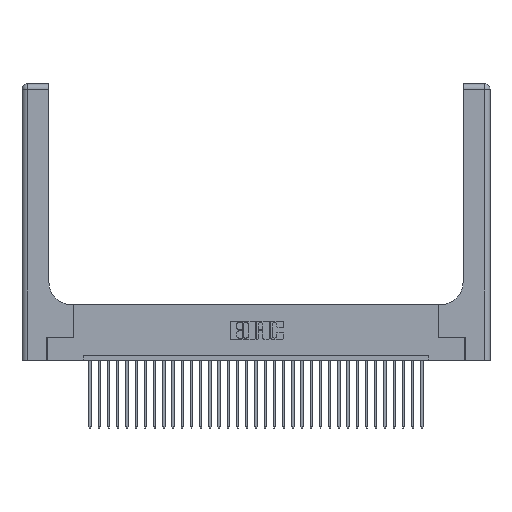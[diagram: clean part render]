
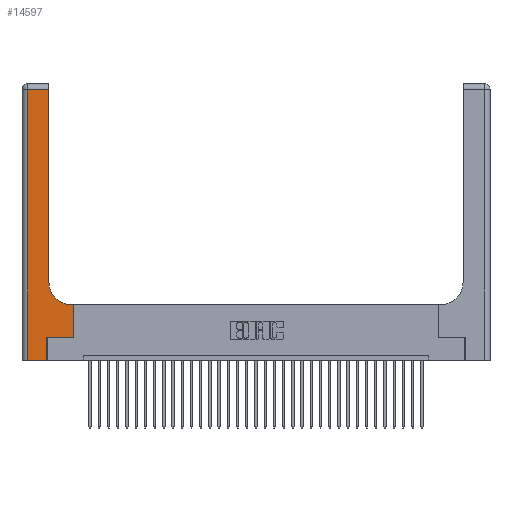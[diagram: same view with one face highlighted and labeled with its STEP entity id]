
A CAD part, top view. The second image highlights one B-rep face of the part: STEP entity #14597.
In plain terms, the highlighted planar face has unit normal (0, 0, 1).
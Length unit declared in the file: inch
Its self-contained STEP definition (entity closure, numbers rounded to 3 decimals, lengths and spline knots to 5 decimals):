
#437 = CARTESIAN_POINT ( 'NONE',  ( 0.2915, 2.94, 0.37 ) ) ;
#638 = LINE ( 'NONE', #29766, #29115 ) ;
#1435 = CARTESIAN_POINT ( 'NONE',  ( 0.269, 0., 0.37 ) ) ;
#1595 = CARTESIAN_POINT ( 'NONE',  ( 0.06, 3., 0.37 ) ) ;
#2507 = CARTESIAN_POINT ( 'NONE',  ( 0.5585, 0.25, 0.37 ) ) ;
#3038 = LINE ( 'NONE', #1595, #9125 ) ;
#3089 = CARTESIAN_POINT ( 'NONE',  ( 0.2915, 0.85, 0.37 ) ) ;
#4243 = CARTESIAN_POINT ( 'NONE',  ( 0., 2.94, 0.37 ) ) ;
#4398 = DIRECTION ( 'NONE',  ( 0., -1., 0. ) ) ;
#4540 = EDGE_CURVE ( 'NONE', #19129, #27300, #638, .T. ) ;
#4602 = CIRCLE ( 'NONE', #20730, 0.25 ) ;
#4735 = ORIENTED_EDGE ( 'NONE', *, *, #5276, .T. ) ;
#4983 = EDGE_CURVE ( 'NONE', #29501, #6721, #3038, .T. ) ;
#5276 = EDGE_CURVE ( 'NONE', #26960, #6509, #13142, .T. ) ;
#5476 = DIRECTION ( 'NONE',  ( 0., 0., -1. ) ) ;
#5525 = EDGE_LOOP ( 'NONE', ( #29854, #11609, #25948, #6923, #5589, #17355, #8979, #4735, #11502 ) ) ;
#5589 = ORIENTED_EDGE ( 'NONE', *, *, #4540, .T. ) ;
#5945 = EDGE_CURVE ( 'NONE', #6509, #29400, #4602, .T. ) ;
#6066 = FACE_OUTER_BOUND ( 'NONE', #5525, .T. ) ;
#6234 = VERTEX_POINT ( 'NONE', #26615 ) ;
#6292 = VECTOR ( 'NONE', #12925, 39.37008 ) ;
#6509 = VERTEX_POINT ( 'NONE', #17719 ) ;
#6721 = VERTEX_POINT ( 'NONE', #9670 ) ;
#6923 = ORIENTED_EDGE ( 'NONE', *, *, #22245, .T. ) ;
#8297 = EDGE_CURVE ( 'NONE', #6234, #26960, #10382, .T. ) ;
#8398 = DIRECTION ( 'NONE',  ( 0., 1., 0. ) ) ;
#8979 = ORIENTED_EDGE ( 'NONE', *, *, #8297, .T. ) ;
#9125 = VECTOR ( 'NONE', #4398, 39.37008 ) ;
#9256 = EDGE_CURVE ( 'NONE', #14236, #29501, #19322, .T. ) ;
#9670 = CARTESIAN_POINT ( 'NONE',  ( 0.06, 0., 0.37 ) ) ;
#10382 = LINE ( 'NONE', #2507, #6292 ) ;
#11502 = ORIENTED_EDGE ( 'NONE', *, *, #5945, .T. ) ;
#11609 = ORIENTED_EDGE ( 'NONE', *, *, #9256, .T. ) ;
#12622 = DIRECTION ( 'NONE',  ( 0., 0., -1. ) ) ;
#12925 = DIRECTION ( 'NONE',  ( 0., 1., 0. ) ) ;
#13142 = LINE ( 'NONE', #13813, #26629 ) ;
#13193 = CARTESIAN_POINT ( 'NONE',  ( 0.5415, 0.85, 0.37 ) ) ;
#13676 = VECTOR ( 'NONE', #24176, 39.37008 ) ;
#13813 = CARTESIAN_POINT ( 'NONE',  ( 0.2915, 0.6, 0.37 ) ) ;
#14236 = VERTEX_POINT ( 'NONE', #437 ) ;
#14381 = EDGE_CURVE ( 'NONE', #27300, #6234, #25894, .T. ) ;
#14403 = VECTOR ( 'NONE', #22439, 39.37008 ) ;
#14597 = ADVANCED_FACE ( 'NONE', ( #6066 ), #28470, .F. ) ;
#14601 = LINE ( 'NONE', #24186, #14990 ) ;
#14990 = VECTOR ( 'NONE', #8398, 39.37008 ) ;
#15243 = CARTESIAN_POINT ( 'NONE',  ( 0., 3., 0.37 ) ) ;
#16738 = CARTESIAN_POINT ( 'NONE',  ( 0.269, 0.25, 0.37 ) ) ;
#17355 = ORIENTED_EDGE ( 'NONE', *, *, #14381, .T. ) ;
#17719 = CARTESIAN_POINT ( 'NONE',  ( 0.5415, 0.6, 0.37 ) ) ;
#18124 = CARTESIAN_POINT ( 'NONE',  ( 0.5585, 0.6, 0.37 ) ) ;
#19129 = VERTEX_POINT ( 'NONE', #1435 ) ;
#19322 = LINE ( 'NONE', #4243, #14403 ) ;
#20063 = DIRECTION ( 'NONE',  ( 1., 0., 0. ) ) ;
#20730 = AXIS2_PLACEMENT_3D ( 'NONE', #13193, #5476, #26065 ) ;
#21368 = DIRECTION ( 'NONE',  ( -1., 0., 0. ) ) ;
#22245 = EDGE_CURVE ( 'NONE', #6721, #19129, #22281, .T. ) ;
#22281 = LINE ( 'NONE', #30429, #27972 ) ;
#22439 = DIRECTION ( 'NONE',  ( -1., 0., 0. ) ) ;
#24176 = DIRECTION ( 'NONE',  ( 1., 0., 0. ) ) ;
#24186 = CARTESIAN_POINT ( 'NONE',  ( 0.2915, 3., 0.37 ) ) ;
#24537 = CARTESIAN_POINT ( 'NONE',  ( 0.06, 2.94, 0.37 ) ) ;
#25894 = LINE ( 'NONE', #16738, #13676 ) ;
#25948 = ORIENTED_EDGE ( 'NONE', *, *, #4983, .T. ) ;
#26065 = DIRECTION ( 'NONE',  ( 1., 0., 0. ) ) ;
#26615 = CARTESIAN_POINT ( 'NONE',  ( 0.5585, 0.25, 0.37 ) ) ;
#26629 = VECTOR ( 'NONE', #21368, 39.37008 ) ;
#26960 = VERTEX_POINT ( 'NONE', #18124 ) ;
#27139 = EDGE_CURVE ( 'NONE', #29400, #14236, #14601, .T. ) ;
#27300 = VERTEX_POINT ( 'NONE', #32299 ) ;
#27652 = AXIS2_PLACEMENT_3D ( 'NONE', #15243, #12622, #31208 ) ;
#27972 = VECTOR ( 'NONE', #20063, 39.37008 ) ;
#28470 = PLANE ( 'NONE',  #27652 ) ;
#29115 = VECTOR ( 'NONE', #29654, 39.37008 ) ;
#29400 = VERTEX_POINT ( 'NONE', #3089 ) ;
#29501 = VERTEX_POINT ( 'NONE', #24537 ) ;
#29654 = DIRECTION ( 'NONE',  ( 0., 1., 0. ) ) ;
#29766 = CARTESIAN_POINT ( 'NONE',  ( 0.269, 0., 0.37 ) ) ;
#29854 = ORIENTED_EDGE ( 'NONE', *, *, #27139, .T. ) ;
#30429 = CARTESIAN_POINT ( 'NONE',  ( 0., 0., 0.37 ) ) ;
#31208 = DIRECTION ( 'NONE',  ( -1., 0., 0. ) ) ;
#32299 = CARTESIAN_POINT ( 'NONE',  ( 0.269, 0.25, 0.37 ) ) ;
